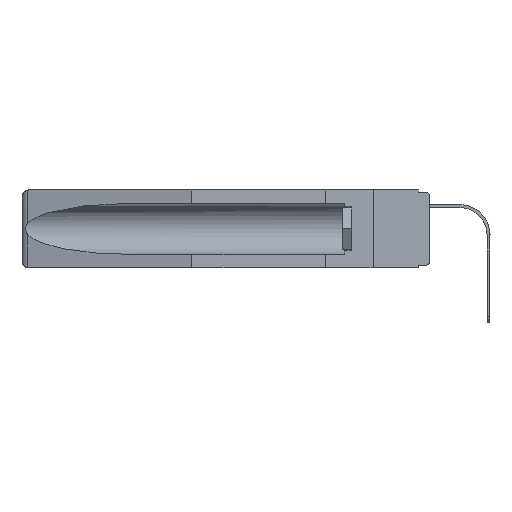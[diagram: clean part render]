
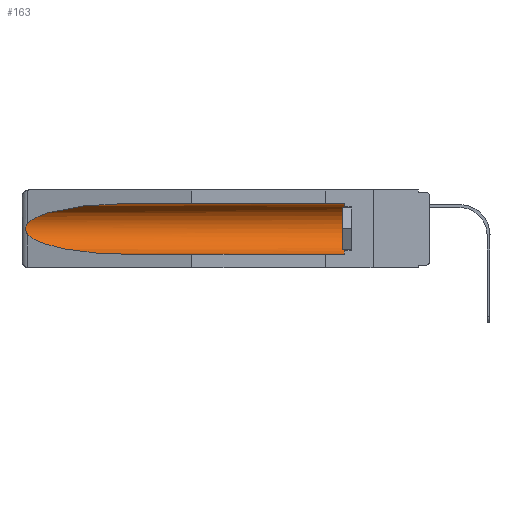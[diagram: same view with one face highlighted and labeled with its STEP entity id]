
A CAD part, left-side view. The second image highlights one B-rep face of the part: STEP entity #163.
In plain terms, the highlighted cylindrical face has radius 2.857 mm (diameter 5.715 mm), a partial arc.
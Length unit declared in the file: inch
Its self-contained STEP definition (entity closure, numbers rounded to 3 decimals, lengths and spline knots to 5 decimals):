
#163 = ADVANCED_FACE ( 'NONE', ( #11921 ), #10890, .F. ) ;
#300 = VECTOR ( 'NONE', #10592, 39.37008 ) ;
#390 = EDGE_CURVE ( 'NONE', #11573, #7777, #3741, .T. ) ;
#581 = EDGE_CURVE ( 'NONE', #11948, #13378, #15024, .T. ) ;
#688 = LINE ( 'NONE', #16119, #1172 ) ;
#703 = CARTESIAN_POINT ( 'NONE',  ( 0.26597, 1.5296, -0.19026 ) ) ;
#1172 = VECTOR ( 'NONE', #11094, 39.37008 ) ;
#1493 = CARTESIAN_POINT ( 'NONE',  ( 0.26537, 1.52718, -0.19328 ) ) ;
#1571 = CARTESIAN_POINT ( 'NONE',  ( 0.21114, 1.30732, -0.284 ) ) ;
#1763 = CARTESIAN_POINT ( 'NONE',  ( 0.155, 0.126, -0.059 ) ) ;
#1835 = CARTESIAN_POINT ( 'NONE',  ( 0.25451, 1.48313, -0.09465 ) ) ;
#2286 = CARTESIAN_POINT ( 'NONE',  ( 0.26537, 1.52718, -0.19328 ) ) ;
#2336 = CARTESIAN_POINT ( 'NONE',  ( 0.26537, 1.52718, -0.14972 ) ) ;
#2824 = CARTESIAN_POINT ( 'NONE',  ( 0.26537, 1.52718, -0.19328 ) ) ;
#3026 = LINE ( 'NONE', #5475, #300 ) ;
#3098 = EDGE_LOOP ( 'NONE', ( #5970, #5943, #13559, #5554, #15028, #10936 ) ) ;
#3411 = CARTESIAN_POINT ( 'NONE',  ( 0.155, 0.126, -0.1715 ) ) ;
#3677 = B_SPLINE_CURVE_WITH_KNOTS ( 'NONE', 3,
 ( #12221, #15053, #16140, #11114, #4556, #16374, #16283, #4654, #703, #2286 ),
 .UNSPECIFIED., .F., .F.,
 ( 4, 2, 2, 2, 4 ),
 ( 0., 0.00029, 0.00058, 0.00087, 0.00117 ),
 .UNSPECIFIED. ) ;
#3741 =( BOUNDED_CURVE ( )  B_SPLINE_CURVE ( 3, ( #13484, #10924, #1835, #7068 ),
 .UNSPECIFIED., .F., .F. ) 
 B_SPLINE_CURVE_WITH_KNOTS ( ( 4, 4 ),
 ( 4.71239, 6.08839 ),
 .UNSPECIFIED. ) 
 CURVE ( )  GEOMETRIC_REPRESENTATION_ITEM ( )  RATIONAL_B_SPLINE_CURVE ( ( 1., 0.848, 0.848, 1. ) ) 
 REPRESENTATION_ITEM ( '' )  );
#4556 = CARTESIAN_POINT ( 'NONE',  ( 0.2675, 1.53308, -0.16763 ) ) ;
#4654 = CARTESIAN_POINT ( 'NONE',  ( 0.26655, 1.53094, -0.18657 ) ) ;
#5156 = CARTESIAN_POINT ( 'NONE',  ( 0.155, 0.126, -0.284 ) ) ;
#5429 = CARTESIAN_POINT ( 'NONE',  ( 0.155, 1.07973, -0.059 ) ) ;
#5475 = CARTESIAN_POINT ( 'NONE',  ( 0.155, -0.30754, -0.059 ) ) ;
#5554 = ORIENTED_EDGE ( 'NONE', *, *, #7686, .F. ) ;
#5943 = ORIENTED_EDGE ( 'NONE', *, *, #5971, .T. ) ;
#5961 = DIRECTION ( 'NONE',  ( 0., 0., 1. ) ) ;
#5970 = ORIENTED_EDGE ( 'NONE', *, *, #390, .T. ) ;
#5971 = EDGE_CURVE ( 'NONE', #7777, #14833, #3677, .T. ) ;
#6193 = AXIS2_PLACEMENT_3D ( 'NONE', #3411, #9654, #5961 ) ;
#6328 = EDGE_CURVE ( 'NONE', #13378, #11573, #3026, .T. ) ;
#7068 = CARTESIAN_POINT ( 'NONE',  ( 0.26537, 1.52718, -0.14972 ) ) ;
#7686 = EDGE_CURVE ( 'NONE', #11948, #8417, #688, .T. ) ;
#7777 = VERTEX_POINT ( 'NONE', #2336 ) ;
#8275 = DIRECTION ( 'NONE',  ( 0., 1., 0. ) ) ;
#8417 = VERTEX_POINT ( 'NONE', #13016 ) ;
#9150 = CARTESIAN_POINT ( 'NONE',  ( 0.155, 1.07973, -0.284 ) ) ;
#9473 = DIRECTION ( 'NONE',  ( 0., 0., 1. ) ) ;
#9654 = DIRECTION ( 'NONE',  ( 0., -1., 0. ) ) ;
#10592 = DIRECTION ( 'NONE',  ( 0., 1., 0. ) ) ;
#10890 = CYLINDRICAL_SURFACE ( 'NONE', #13948, 0.1125 ) ;
#10924 = CARTESIAN_POINT ( 'NONE',  ( 0.21114, 1.30732, -0.059 ) ) ;
#10936 = ORIENTED_EDGE ( 'NONE', *, *, #6328, .T. ) ;
#11094 = DIRECTION ( 'NONE',  ( 0., 1., 0. ) ) ;
#11114 = CARTESIAN_POINT ( 'NONE',  ( 0.2673, 1.5327, -0.16383 ) ) ;
#11573 = VERTEX_POINT ( 'NONE', #5429 ) ;
#11921 = FACE_OUTER_BOUND ( 'NONE', #3098, .T. ) ;
#11948 = VERTEX_POINT ( 'NONE', #5156 ) ;
#12221 = CARTESIAN_POINT ( 'NONE',  ( 0.26537, 1.52718, -0.14972 ) ) ;
#12731 = CARTESIAN_POINT ( 'NONE',  ( 0.25451, 1.48313, -0.24835 ) ) ;
#13016 = CARTESIAN_POINT ( 'NONE',  ( 0.155, 1.07973, -0.284 ) ) ;
#13378 = VERTEX_POINT ( 'NONE', #1763 ) ;
#13484 = CARTESIAN_POINT ( 'NONE',  ( 0.155, 1.07973, -0.059 ) ) ;
#13546 =( BOUNDED_CURVE ( )  B_SPLINE_CURVE ( 3, ( #1493, #12731, #1571, #9150 ),
 .UNSPECIFIED., .F., .F. ) 
 B_SPLINE_CURVE_WITH_KNOTS ( ( 4, 4 ),
 ( 0.1948, 1.5708 ),
 .UNSPECIFIED. ) 
 CURVE ( )  GEOMETRIC_REPRESENTATION_ITEM ( )  RATIONAL_B_SPLINE_CURVE ( ( 1., 0.848, 0.848, 1. ) ) 
 REPRESENTATION_ITEM ( '' )  );
#13559 = ORIENTED_EDGE ( 'NONE', *, *, #14396, .T. ) ;
#13948 = AXIS2_PLACEMENT_3D ( 'NONE', #16008, #8275, #9473 ) ;
#14396 = EDGE_CURVE ( 'NONE', #14833, #8417, #13546, .T. ) ;
#14833 = VERTEX_POINT ( 'NONE', #2824 ) ;
#15024 = CIRCLE ( 'NONE', #6193, 0.1125 ) ;
#15028 = ORIENTED_EDGE ( 'NONE', *, *, #581, .T. ) ;
#15053 = CARTESIAN_POINT ( 'NONE',  ( 0.26597, 1.52961, -0.15275 ) ) ;
#16008 = CARTESIAN_POINT ( 'NONE',  ( 0.155, -0.30754, -0.1715 ) ) ;
#16119 = CARTESIAN_POINT ( 'NONE',  ( 0.155, -0.30754, -0.284 ) ) ;
#16140 = CARTESIAN_POINT ( 'NONE',  ( 0.26654, 1.53092, -0.15636 ) ) ;
#16283 = CARTESIAN_POINT ( 'NONE',  ( 0.2673, 1.53269, -0.17917 ) ) ;
#16374 = CARTESIAN_POINT ( 'NONE',  ( 0.2675, 1.53308, -0.17534 ) ) ;
